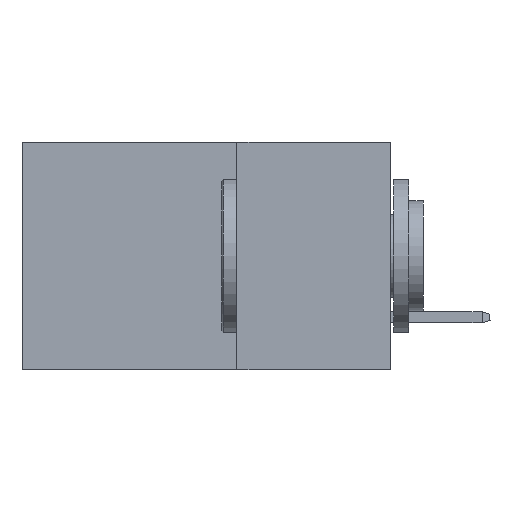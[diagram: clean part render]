
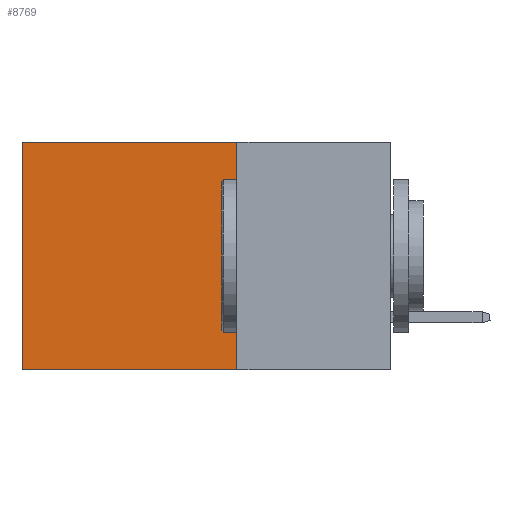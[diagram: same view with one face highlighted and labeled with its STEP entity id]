
A CAD part, left-side view. The second image highlights one B-rep face of the part: STEP entity #8769.
In plain terms, the highlighted planar face has unit normal (-1, 0, 0).
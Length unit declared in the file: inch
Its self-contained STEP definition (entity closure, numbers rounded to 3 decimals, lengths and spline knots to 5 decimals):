
#131 = CARTESIAN_POINT ( 'NONE',  ( 0.2875, 0.25, 0. ) ) ;
#318 = CARTESIAN_POINT ( 'NONE',  ( 0.2875, 0.25, 0. ) ) ;
#727 = VERTEX_POINT ( 'NONE', #22321 ) ;
#1745 = CARTESIAN_POINT ( 'NONE',  ( 0.2875, 0.6, 0. ) ) ;
#2171 = DIRECTION ( 'NONE',  ( 0., 0., -1. ) ) ;
#3025 = PLANE ( 'NONE',  #21825 ) ;
#3645 = VERTEX_POINT ( 'NONE', #318 ) ;
#4065 = VECTOR ( 'NONE', #2171, 39.37008 ) ;
#4816 = EDGE_CURVE ( 'NONE', #3645, #15835, #8666, .T. ) ;
#4932 = CARTESIAN_POINT ( 'NONE',  ( 0.2875, 0.25, 0. ) ) ;
#5255 = LINE ( 'NONE', #11079, #14208 ) ;
#5744 = EDGE_CURVE ( 'NONE', #15835, #727, #11849, .T. ) ;
#6681 = DIRECTION ( 'NONE',  ( 1., 0., 0. ) ) ;
#6711 = ORIENTED_EDGE ( 'NONE', *, *, #8638, .T. ) ;
#7123 = CARTESIAN_POINT ( 'NONE',  ( 0.2875, 0.6, 0. ) ) ;
#7318 = VECTOR ( 'NONE', #17628, 39.37008 ) ;
#8002 = CARTESIAN_POINT ( 'NONE',  ( 0.2875, 0.25, -0.37 ) ) ;
#8638 = EDGE_CURVE ( 'NONE', #3645, #14736, #5255, .T. ) ;
#8666 = LINE ( 'NONE', #131, #4065 ) ;
#8705 = ORIENTED_EDGE ( 'NONE', *, *, #12597, .T. ) ;
#8769 = ADVANCED_FACE ( 'NONE', ( #15547 ), #3025, .F. ) ;
#9230 = ORIENTED_EDGE ( 'NONE', *, *, #5744, .F. ) ;
#9886 = CARTESIAN_POINT ( 'NONE',  ( 0.2875, 0.25, -0.37 ) ) ;
#11079 = CARTESIAN_POINT ( 'NONE',  ( 0.2875, 0.25, 0. ) ) ;
#11574 = DIRECTION ( 'NONE',  ( 0., 1., 0. ) ) ;
#11849 = LINE ( 'NONE', #8002, #13192 ) ;
#12485 = LINE ( 'NONE', #7123, #7318 ) ;
#12597 = EDGE_CURVE ( 'NONE', #14736, #727, #12485, .T. ) ;
#13192 = VECTOR ( 'NONE', #11574, 39.37008 ) ;
#14208 = VECTOR ( 'NONE', #18075, 39.37008 ) ;
#14736 = VERTEX_POINT ( 'NONE', #1745 ) ;
#15312 = DIRECTION ( 'NONE',  ( 0., 0., -1. ) ) ;
#15547 = FACE_OUTER_BOUND ( 'NONE', #19754, .T. ) ;
#15557 = ORIENTED_EDGE ( 'NONE', *, *, #4816, .F. ) ;
#15835 = VERTEX_POINT ( 'NONE', #9886 ) ;
#17628 = DIRECTION ( 'NONE',  ( 0., 0., -1. ) ) ;
#18075 = DIRECTION ( 'NONE',  ( 0., 1., 0. ) ) ;
#19754 = EDGE_LOOP ( 'NONE', ( #8705, #9230, #15557, #6711 ) ) ;
#21825 = AXIS2_PLACEMENT_3D ( 'NONE', #4932, #6681, #15312 ) ;
#22321 = CARTESIAN_POINT ( 'NONE',  ( 0.2875, 0.6, -0.37 ) ) ;
